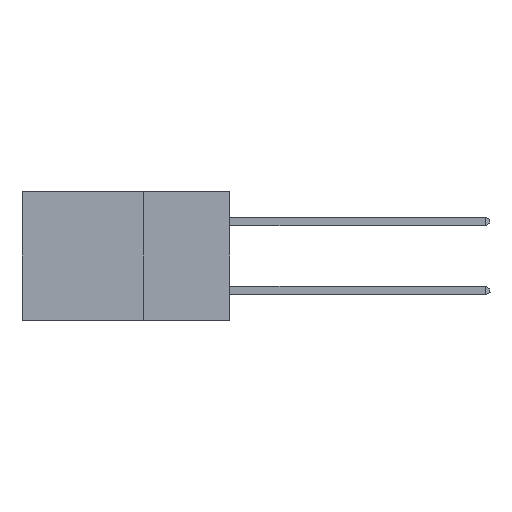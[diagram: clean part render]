
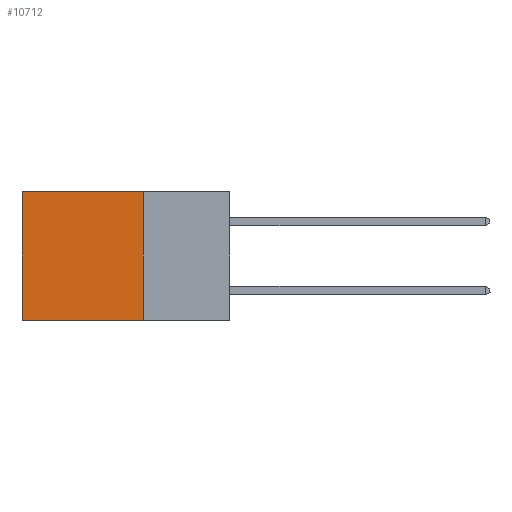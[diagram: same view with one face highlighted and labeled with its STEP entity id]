
A CAD part, left-side view. The second image highlights one B-rep face of the part: STEP entity #10712.
In plain terms, the highlighted planar face has unit normal (-1, 0, 0).
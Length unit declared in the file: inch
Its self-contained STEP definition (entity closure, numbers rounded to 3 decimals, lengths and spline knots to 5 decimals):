
#244 = VERTEX_POINT ( 'NONE', #11651 ) ;
#507 = ORIENTED_EDGE ( 'NONE', *, *, #2471, .T. ) ;
#937 = EDGE_CURVE ( 'NONE', #12090, #10492, #4669, .T. ) ;
#972 = DIRECTION ( 'NONE',  ( 0., 1., 0. ) ) ;
#987 = VECTOR ( 'NONE', #6022, 39.37008 ) ;
#1026 = EDGE_CURVE ( 'NONE', #12090, #6969, #11478, .T. ) ;
#1615 = CARTESIAN_POINT ( 'NONE',  ( 0.298, 0.25, 0. ) ) ;
#1829 = CARTESIAN_POINT ( 'NONE',  ( 0.298, 0.25, 0. ) ) ;
#2471 = EDGE_CURVE ( 'NONE', #6969, #244, #7129, .T. ) ;
#2661 = DIRECTION ( 'NONE',  ( 0., 0., -1. ) ) ;
#2977 = CARTESIAN_POINT ( 'NONE',  ( 0.298, 0.6, 0. ) ) ;
#3082 = FACE_OUTER_BOUND ( 'NONE', #10010, .T. ) ;
#3457 = VECTOR ( 'NONE', #972, 39.37008 ) ;
#3670 = CARTESIAN_POINT ( 'NONE',  ( 0.298, 0.6, 0. ) ) ;
#4353 = PLANE ( 'NONE',  #12019 ) ;
#4381 = VECTOR ( 'NONE', #2661, 39.37008 ) ;
#4669 = LINE ( 'NONE', #1829, #4381 ) ;
#4995 = ORIENTED_EDGE ( 'NONE', *, *, #11941, .F. ) ;
#6022 = DIRECTION ( 'NONE',  ( 0., 1., 0. ) ) ;
#6969 = VERTEX_POINT ( 'NONE', #3670 ) ;
#7083 = CARTESIAN_POINT ( 'NONE',  ( 0.298, 0.25, -0.37 ) ) ;
#7129 = LINE ( 'NONE', #2977, #7264 ) ;
#7264 = VECTOR ( 'NONE', #9590, 39.37008 ) ;
#8160 = ORIENTED_EDGE ( 'NONE', *, *, #937, .F. ) ;
#8177 = DIRECTION ( 'NONE',  ( 1., 0., 0. ) ) ;
#8852 = CARTESIAN_POINT ( 'NONE',  ( 0.298, 0.25, 0. ) ) ;
#8920 = ORIENTED_EDGE ( 'NONE', *, *, #1026, .T. ) ;
#9253 = LINE ( 'NONE', #7083, #987 ) ;
#9590 = DIRECTION ( 'NONE',  ( 0., 0., -1. ) ) ;
#10010 = EDGE_LOOP ( 'NONE', ( #507, #4995, #8160, #8920 ) ) ;
#10492 = VERTEX_POINT ( 'NONE', #11374 ) ;
#10712 = ADVANCED_FACE ( 'NONE', ( #3082 ), #4353, .F. ) ;
#11374 = CARTESIAN_POINT ( 'NONE',  ( 0.298, 0.25, -0.37 ) ) ;
#11478 = LINE ( 'NONE', #12245, #3457 ) ;
#11651 = CARTESIAN_POINT ( 'NONE',  ( 0.298, 0.6, -0.37 ) ) ;
#11941 = EDGE_CURVE ( 'NONE', #10492, #244, #9253, .T. ) ;
#12019 = AXIS2_PLACEMENT_3D ( 'NONE', #1615, #8177, #12039 ) ;
#12039 = DIRECTION ( 'NONE',  ( 0., 0., -1. ) ) ;
#12090 = VERTEX_POINT ( 'NONE', #8852 ) ;
#12245 = CARTESIAN_POINT ( 'NONE',  ( 0.298, 0.25, 0. ) ) ;
